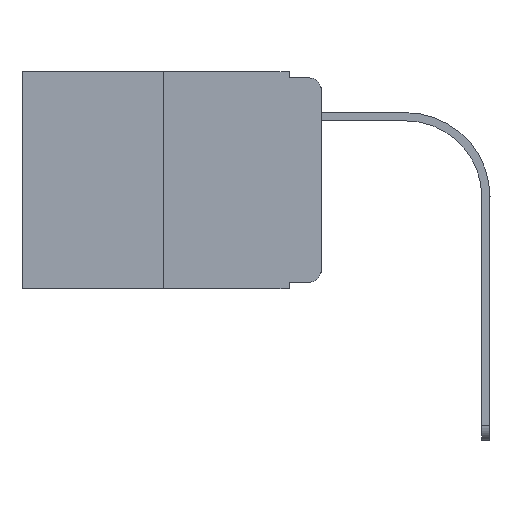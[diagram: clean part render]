
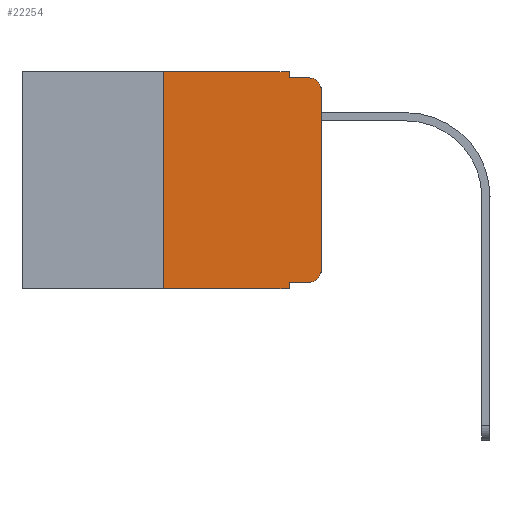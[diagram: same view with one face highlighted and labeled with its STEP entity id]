
A CAD part, left-side view. The second image highlights one B-rep face of the part: STEP entity #22254.
In plain terms, the highlighted planar face has unit normal (-1, 0, 0).
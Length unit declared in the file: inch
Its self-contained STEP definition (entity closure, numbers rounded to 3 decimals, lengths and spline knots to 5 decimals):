
#182 = LINE ( 'NONE', #14648, #10203 ) ;
#521 = VERTEX_POINT ( 'NONE', #17972 ) ;
#538 = CARTESIAN_POINT ( 'NONE',  ( 0., 0.02, -0.333 ) ) ;
#1157 = CARTESIAN_POINT ( 'NONE',  ( 0., 0.051, 0. ) ) ;
#1268 = EDGE_CURVE ( 'NONE', #17225, #7181, #19481, .T. ) ;
#1338 = ORIENTED_EDGE ( 'NONE', *, *, #6833, .T. ) ;
#2040 = CARTESIAN_POINT ( 'NONE',  ( 0., 0.051, -0.01 ) ) ;
#2130 = EDGE_CURVE ( 'NONE', #521, #5800, #22481, .T. ) ;
#2462 = DIRECTION ( 'NONE',  ( 0., -1., 0. ) ) ;
#2503 = CARTESIAN_POINT ( 'NONE',  ( 0., 0.02, -0.01 ) ) ;
#3579 = ORIENTED_EDGE ( 'NONE', *, *, #5216, .F. ) ;
#3599 = EDGE_CURVE ( 'NONE', #9317, #16421, #4888, .T. ) ;
#3607 = ORIENTED_EDGE ( 'NONE', *, *, #7823, .T. ) ;
#3792 = ORIENTED_EDGE ( 'NONE', *, *, #7853, .T. ) ;
#3827 = DIRECTION ( 'NONE',  ( 0., 0., 1. ) ) ;
#4155 = DIRECTION ( 'NONE',  ( -1., 0., 0. ) ) ;
#4216 = EDGE_LOOP ( 'NONE', ( #1338, #19116, #22780, #7933, #3579, #7339, #3792, #5031, #3607, #9924 ) ) ;
#4309 = VERTEX_POINT ( 'NONE', #9809 ) ;
#4408 = VERTEX_POINT ( 'NONE', #6490 ) ;
#4640 = DIRECTION ( 'NONE',  ( 0., 0., -1. ) ) ;
#4857 = FACE_OUTER_BOUND ( 'NONE', #4216, .T. ) ;
#4888 = LINE ( 'NONE', #15729, #5662 ) ;
#5031 = ORIENTED_EDGE ( 'NONE', *, *, #18284, .F. ) ;
#5216 = EDGE_CURVE ( 'NONE', #4408, #9317, #13464, .T. ) ;
#5600 = VECTOR ( 'NONE', #18167, 39.37008 ) ;
#5662 = VECTOR ( 'NONE', #22879, 39.37008 ) ;
#5798 = DIRECTION ( 'NONE',  ( -1., 0., 0. ) ) ;
#5800 = VERTEX_POINT ( 'NONE', #2503 ) ;
#5885 = LINE ( 'NONE', #15295, #12973 ) ;
#6490 = CARTESIAN_POINT ( 'NONE',  ( 0., 0.25, 0. ) ) ;
#6833 = EDGE_CURVE ( 'NONE', #7181, #521, #19377, .T. ) ;
#6922 = LINE ( 'NONE', #2040, #5600 ) ;
#7181 = VERTEX_POINT ( 'NONE', #15222 ) ;
#7339 = ORIENTED_EDGE ( 'NONE', *, *, #8198, .F. ) ;
#7823 = EDGE_CURVE ( 'NONE', #15961, #17225, #16586, .T. ) ;
#7853 = EDGE_CURVE ( 'NONE', #22021, #4309, #5885, .T. ) ;
#7933 = ORIENTED_EDGE ( 'NONE', *, *, #3599, .F. ) ;
#8099 = CARTESIAN_POINT ( 'NONE',  ( 0., 0.051, -0.01 ) ) ;
#8198 = EDGE_CURVE ( 'NONE', #22021, #4408, #182, .T. ) ;
#8216 = CARTESIAN_POINT ( 'NONE',  ( 0., 0.02, -0.03 ) ) ;
#8532 = AXIS2_PLACEMENT_3D ( 'NONE', #8216, #4155, #4640 ) ;
#9317 = VERTEX_POINT ( 'NONE', #1157 ) ;
#9809 = CARTESIAN_POINT ( 'NONE',  ( 0., 0.051, -0.343 ) ) ;
#9924 = ORIENTED_EDGE ( 'NONE', *, *, #1268, .T. ) ;
#10203 = VECTOR ( 'NONE', #3827, 39.37008 ) ;
#10240 = CARTESIAN_POINT ( 'NONE',  ( 0., 0.051, -0.333 ) ) ;
#11395 = CARTESIAN_POINT ( 'NONE',  ( 0., 0.02, -0.313 ) ) ;
#11662 = DIRECTION ( 'NONE',  ( 1., 0., 0. ) ) ;
#12587 = VECTOR ( 'NONE', #13154, 39.37008 ) ;
#12973 = VECTOR ( 'NONE', #2462, 39.37008 ) ;
#13154 = DIRECTION ( 'NONE',  ( 0., -1., 0. ) ) ;
#13214 = DIRECTION ( 'NONE',  ( 0., -1., 0. ) ) ;
#13464 = LINE ( 'NONE', #22174, #14792 ) ;
#14648 = CARTESIAN_POINT ( 'NONE',  ( 0., 0.25, 0. ) ) ;
#14792 = VECTOR ( 'NONE', #13214, 39.37008 ) ;
#15222 = CARTESIAN_POINT ( 'NONE',  ( 0., 0., -0.313 ) ) ;
#15295 = CARTESIAN_POINT ( 'NONE',  ( 0., 0.473, -0.343 ) ) ;
#15702 = PLANE ( 'NONE',  #18219 ) ;
#15729 = CARTESIAN_POINT ( 'NONE',  ( 0., 0.051, 0. ) ) ;
#15816 = CARTESIAN_POINT ( 'NONE',  ( 0., 0.051, 0. ) ) ;
#15961 = VERTEX_POINT ( 'NONE', #10240 ) ;
#16421 = VERTEX_POINT ( 'NONE', #8099 ) ;
#16586 = LINE ( 'NONE', #22342, #12587 ) ;
#17225 = VERTEX_POINT ( 'NONE', #538 ) ;
#17233 = AXIS2_PLACEMENT_3D ( 'NONE', #11395, #5798, #22025 ) ;
#17724 = DIRECTION ( 'NONE',  ( 0., 0., 1. ) ) ;
#17972 = CARTESIAN_POINT ( 'NONE',  ( 0., 0., -0.03 ) ) ;
#18167 = DIRECTION ( 'NONE',  ( 0., -1., 0. ) ) ;
#18219 = AXIS2_PLACEMENT_3D ( 'NONE', #21082, #11662, #22748 ) ;
#18284 = EDGE_CURVE ( 'NONE', #15961, #4309, #21095, .T. ) ;
#18376 = EDGE_CURVE ( 'NONE', #16421, #5800, #6922, .T. ) ;
#18543 = VECTOR ( 'NONE', #20752, 39.37008 ) ;
#19116 = ORIENTED_EDGE ( 'NONE', *, *, #2130, .T. ) ;
#19377 = LINE ( 'NONE', #20999, #21137 ) ;
#19481 = CIRCLE ( 'NONE', #17233, 0.02 ) ;
#20168 = CARTESIAN_POINT ( 'NONE',  ( 0., 0.25, -0.343 ) ) ;
#20752 = DIRECTION ( 'NONE',  ( 0., 0., -1. ) ) ;
#20999 = CARTESIAN_POINT ( 'NONE',  ( 0., 0., 0. ) ) ;
#21082 = CARTESIAN_POINT ( 'NONE',  ( 0., 0.473, 0. ) ) ;
#21095 = LINE ( 'NONE', #15816, #18543 ) ;
#21137 = VECTOR ( 'NONE', #17724, 39.37008 ) ;
#22021 = VERTEX_POINT ( 'NONE', #20168 ) ;
#22025 = DIRECTION ( 'NONE',  ( 0., 0., -1. ) ) ;
#22174 = CARTESIAN_POINT ( 'NONE',  ( 0., 0.473, 0. ) ) ;
#22254 = ADVANCED_FACE ( 'NONE', ( #4857 ), #15702, .F. ) ;
#22342 = CARTESIAN_POINT ( 'NONE',  ( 0., 0.051, -0.333 ) ) ;
#22481 = CIRCLE ( 'NONE', #8532, 0.02 ) ;
#22748 = DIRECTION ( 'NONE',  ( 0., 0., -1. ) ) ;
#22780 = ORIENTED_EDGE ( 'NONE', *, *, #18376, .F. ) ;
#22879 = DIRECTION ( 'NONE',  ( 0., 0., -1. ) ) ;
